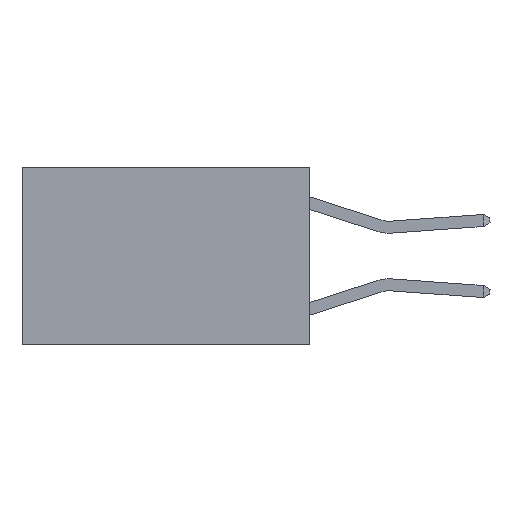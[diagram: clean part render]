
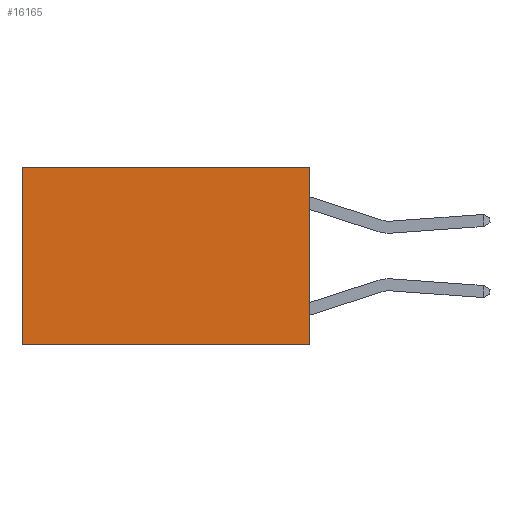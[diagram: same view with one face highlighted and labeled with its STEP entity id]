
A CAD part, left-side view. The second image highlights one B-rep face of the part: STEP entity #16165.
In plain terms, the highlighted planar face has unit normal (-1, 0, 0).
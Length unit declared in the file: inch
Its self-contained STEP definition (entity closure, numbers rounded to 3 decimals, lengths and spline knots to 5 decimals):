
#903 = DIRECTION ( 'NONE',  ( 0., 1., 0. ) ) ;
#929 = CARTESIAN_POINT ( 'NONE',  ( 0.2625, 0., -0.37 ) ) ;
#1032 = ORIENTED_EDGE ( 'NONE', *, *, #9200, .F. ) ;
#1106 = DIRECTION ( 'NONE',  ( 0., 0., -1. ) ) ;
#1151 = LINE ( 'NONE', #11362, #15634 ) ;
#1798 = PLANE ( 'NONE',  #10263 ) ;
#1827 = ORIENTED_EDGE ( 'NONE', *, *, #9204, .F. ) ;
#2040 = DIRECTION ( 'NONE',  ( 0., 1., 0. ) ) ;
#2637 = DIRECTION ( 'NONE',  ( 0., 0., -1. ) ) ;
#3731 = CARTESIAN_POINT ( 'NONE',  ( 0.2625, 0.6, 0. ) ) ;
#4692 = EDGE_CURVE ( 'NONE', #14955, #22516, #9976, .T. ) ;
#5306 = CARTESIAN_POINT ( 'NONE',  ( 0.2625, 0., 0. ) ) ;
#5785 = LINE ( 'NONE', #13018, #14536 ) ;
#5845 = VECTOR ( 'NONE', #2040, 39.37008 ) ;
#6218 = LINE ( 'NONE', #21991, #14976 ) ;
#6633 = VERTEX_POINT ( 'NONE', #929 ) ;
#7729 = ORIENTED_EDGE ( 'NONE', *, *, #4692, .T. ) ;
#8845 = DIRECTION ( 'NONE',  ( 1., 0., 0. ) ) ;
#9200 = EDGE_CURVE ( 'NONE', #6633, #19637, #1151, .T. ) ;
#9204 = EDGE_CURVE ( 'NONE', #14955, #6633, #5785, .T. ) ;
#9306 = CARTESIAN_POINT ( 'NONE',  ( 0.2625, 0.6, -0.37 ) ) ;
#9976 = LINE ( 'NONE', #21186, #5845 ) ;
#10263 = AXIS2_PLACEMENT_3D ( 'NONE', #5306, #8845, #21035 ) ;
#11362 = CARTESIAN_POINT ( 'NONE',  ( 0.2625, 0., -0.37 ) ) ;
#13018 = CARTESIAN_POINT ( 'NONE',  ( 0.2625, 0., 0. ) ) ;
#14536 = VECTOR ( 'NONE', #2637, 39.37008 ) ;
#14955 = VERTEX_POINT ( 'NONE', #15849 ) ;
#14976 = VECTOR ( 'NONE', #1106, 39.37008 ) ;
#15634 = VECTOR ( 'NONE', #903, 39.37008 ) ;
#15849 = CARTESIAN_POINT ( 'NONE',  ( 0.2625, 0., 0. ) ) ;
#16165 = ADVANCED_FACE ( 'NONE', ( #21331 ), #1798, .F. ) ;
#16575 = EDGE_LOOP ( 'NONE', ( #19860, #1032, #1827, #7729 ) ) ;
#19637 = VERTEX_POINT ( 'NONE', #9306 ) ;
#19853 = EDGE_CURVE ( 'NONE', #22516, #19637, #6218, .T. ) ;
#19860 = ORIENTED_EDGE ( 'NONE', *, *, #19853, .T. ) ;
#21035 = DIRECTION ( 'NONE',  ( 0., 0., -1. ) ) ;
#21186 = CARTESIAN_POINT ( 'NONE',  ( 0.2625, 0., 0. ) ) ;
#21331 = FACE_OUTER_BOUND ( 'NONE', #16575, .T. ) ;
#21991 = CARTESIAN_POINT ( 'NONE',  ( 0.2625, 0.6, 0. ) ) ;
#22516 = VERTEX_POINT ( 'NONE', #3731 ) ;
